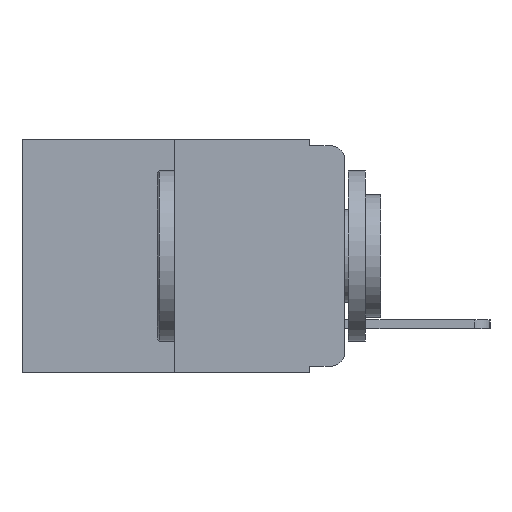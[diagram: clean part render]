
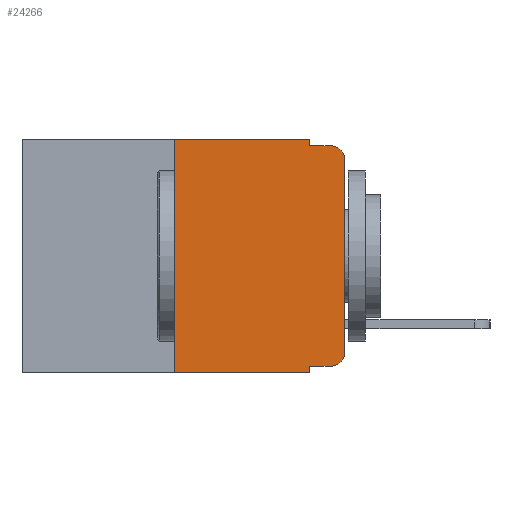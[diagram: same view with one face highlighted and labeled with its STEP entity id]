
A CAD part, left-side view. The second image highlights one B-rep face of the part: STEP entity #24266.
In plain terms, the highlighted planar face has unit normal (-1, 0, 0).
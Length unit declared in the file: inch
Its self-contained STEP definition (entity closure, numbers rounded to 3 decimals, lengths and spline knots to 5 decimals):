
#91 = DIRECTION ( 'NONE',  ( 0., 0., -1. ) ) ;
#935 = VERTEX_POINT ( 'NONE', #13057 ) ;
#1769 = CIRCLE ( 'NONE', #21188, 0.02 ) ;
#1805 = VERTEX_POINT ( 'NONE', #11658 ) ;
#1842 = CARTESIAN_POINT ( 'NONE',  ( 0., 0.051, 0. ) ) ;
#1958 = CARTESIAN_POINT ( 'NONE',  ( 0., 0., -0.03 ) ) ;
#2430 = CARTESIAN_POINT ( 'NONE',  ( 0., 0.473, 0. ) ) ;
#2524 = DIRECTION ( 'NONE',  ( -1., 0., 0. ) ) ;
#2760 = CARTESIAN_POINT ( 'NONE',  ( 0., 0.051, -0.343 ) ) ;
#3143 = CARTESIAN_POINT ( 'NONE',  ( 0., 0.25, -0.343 ) ) ;
#3428 = DIRECTION ( 'NONE',  ( 0., -1., 0. ) ) ;
#3642 = FACE_OUTER_BOUND ( 'NONE', #5323, .T. ) ;
#4246 = VECTOR ( 'NONE', #15215, 39.37008 ) ;
#4511 = VECTOR ( 'NONE', #8944, 39.37008 ) ;
#5126 = CARTESIAN_POINT ( 'NONE',  ( 0., 0.25, 0. ) ) ;
#5323 = EDGE_LOOP ( 'NONE', ( #5848, #6630, #7148, #7383, #7730, #7857, #8048, #8886, #10385, #14913 ) ) ;
#5848 = ORIENTED_EDGE ( 'NONE', *, *, #20655, .T. ) ;
#6630 = ORIENTED_EDGE ( 'NONE', *, *, #19411, .T. ) ;
#6721 = VERTEX_POINT ( 'NONE', #14300 ) ;
#6973 = VECTOR ( 'NONE', #20878, 39.37008 ) ;
#7148 = ORIENTED_EDGE ( 'NONE', *, *, #18197, .F. ) ;
#7259 = EDGE_CURVE ( 'NONE', #7272, #22454, #15063, .T. ) ;
#7272 = VERTEX_POINT ( 'NONE', #3143 ) ;
#7383 = ORIENTED_EDGE ( 'NONE', *, *, #15744, .F. ) ;
#7730 = ORIENTED_EDGE ( 'NONE', *, *, #13868, .F. ) ;
#7857 = ORIENTED_EDGE ( 'NONE', *, *, #14480, .F. ) ;
#7949 = AXIS2_PLACEMENT_3D ( 'NONE', #22651, #11613, #91 ) ;
#8048 = ORIENTED_EDGE ( 'NONE', *, *, #7259, .T. ) ;
#8066 = CARTESIAN_POINT ( 'NONE',  ( 0., 0., -0.313 ) ) ;
#8886 = ORIENTED_EDGE ( 'NONE', *, *, #13232, .F. ) ;
#8944 = DIRECTION ( 'NONE',  ( 0., 0., 1. ) ) ;
#9014 = VERTEX_POINT ( 'NONE', #8066 ) ;
#9462 = VERTEX_POINT ( 'NONE', #1958 ) ;
#9473 = EDGE_CURVE ( 'NONE', #12463, #9014, #19847, .T. ) ;
#9792 = CARTESIAN_POINT ( 'NONE',  ( 0., 0., 0. ) ) ;
#10176 = DIRECTION ( 'NONE',  ( 1., 0., 0. ) ) ;
#10378 = DIRECTION ( 'NONE',  ( 0., -1., 0. ) ) ;
#10385 = ORIENTED_EDGE ( 'NONE', *, *, #10762, .T. ) ;
#10762 = EDGE_CURVE ( 'NONE', #935, #12463, #19188, .T. ) ;
#11473 = CARTESIAN_POINT ( 'NONE',  ( 0., 0.473, 0. ) ) ;
#11613 = DIRECTION ( 'NONE',  ( -1., 0., 0. ) ) ;
#11658 = CARTESIAN_POINT ( 'NONE',  ( 0., 0.25, 0. ) ) ;
#12463 = VERTEX_POINT ( 'NONE', #14345 ) ;
#13057 = CARTESIAN_POINT ( 'NONE',  ( 0., 0.051, -0.333 ) ) ;
#13232 = EDGE_CURVE ( 'NONE', #935, #22454, #22925, .T. ) ;
#13436 = VERTEX_POINT ( 'NONE', #23091 ) ;
#13695 = VECTOR ( 'NONE', #17021, 39.37008 ) ;
#13868 = EDGE_CURVE ( 'NONE', #1805, #6721, #18611, .T. ) ;
#13925 = CARTESIAN_POINT ( 'NONE',  ( 0., 0.02, -0.03 ) ) ;
#14300 = CARTESIAN_POINT ( 'NONE',  ( 0., 0.051, 0. ) ) ;
#14345 = CARTESIAN_POINT ( 'NONE',  ( 0., 0.02, -0.333 ) ) ;
#14480 = EDGE_CURVE ( 'NONE', #7272, #1805, #19436, .T. ) ;
#14913 = ORIENTED_EDGE ( 'NONE', *, *, #9473, .T. ) ;
#15063 = LINE ( 'NONE', #23272, #19374 ) ;
#15215 = DIRECTION ( 'NONE',  ( 0., -1., 0. ) ) ;
#15744 = EDGE_CURVE ( 'NONE', #6721, #13436, #21656, .T. ) ;
#15809 = DIRECTION ( 'NONE',  ( 0., 0., -1. ) ) ;
#16168 = DIRECTION ( 'NONE',  ( 0., 0., -1. ) ) ;
#16659 = CARTESIAN_POINT ( 'NONE',  ( 0., 0.051, -0.01 ) ) ;
#17021 = DIRECTION ( 'NONE',  ( 0., 0., -1. ) ) ;
#17603 = CARTESIAN_POINT ( 'NONE',  ( 0., 0.02, -0.01 ) ) ;
#17934 = VECTOR ( 'NONE', #16168, 39.37008 ) ;
#18012 = CARTESIAN_POINT ( 'NONE',  ( 0., 0.051, 0. ) ) ;
#18052 = VECTOR ( 'NONE', #22502, 39.37008 ) ;
#18197 = EDGE_CURVE ( 'NONE', #13436, #18527, #19541, .T. ) ;
#18527 = VERTEX_POINT ( 'NONE', #17603 ) ;
#18611 = LINE ( 'NONE', #11473, #18052 ) ;
#18990 = AXIS2_PLACEMENT_3D ( 'NONE', #2430, #10176, #23079 ) ;
#19188 = LINE ( 'NONE', #22514, #4246 ) ;
#19374 = VECTOR ( 'NONE', #10378, 39.37008 ) ;
#19411 = EDGE_CURVE ( 'NONE', #9462, #18527, #1769, .T. ) ;
#19436 = LINE ( 'NONE', #5126, #4511 ) ;
#19541 = LINE ( 'NONE', #16659, #20119 ) ;
#19847 = CIRCLE ( 'NONE', #7949, 0.02 ) ;
#20119 = VECTOR ( 'NONE', #3428, 39.37008 ) ;
#20655 = EDGE_CURVE ( 'NONE', #9014, #9462, #21816, .T. ) ;
#20878 = DIRECTION ( 'NONE',  ( 0., 0., 1. ) ) ;
#21188 = AXIS2_PLACEMENT_3D ( 'NONE', #13925, #2524, #15809 ) ;
#21243 = PLANE ( 'NONE',  #18990 ) ;
#21656 = LINE ( 'NONE', #18012, #17934 ) ;
#21816 = LINE ( 'NONE', #9792, #6973 ) ;
#22454 = VERTEX_POINT ( 'NONE', #2760 ) ;
#22502 = DIRECTION ( 'NONE',  ( 0., -1., 0. ) ) ;
#22514 = CARTESIAN_POINT ( 'NONE',  ( 0., 0.051, -0.333 ) ) ;
#22651 = CARTESIAN_POINT ( 'NONE',  ( 0., 0.02, -0.313 ) ) ;
#22925 = LINE ( 'NONE', #1842, #13695 ) ;
#23079 = DIRECTION ( 'NONE',  ( 0., 0., -1. ) ) ;
#23091 = CARTESIAN_POINT ( 'NONE',  ( 0., 0.051, -0.01 ) ) ;
#23272 = CARTESIAN_POINT ( 'NONE',  ( 0., 0.473, -0.343 ) ) ;
#24266 = ADVANCED_FACE ( 'NONE', ( #3642 ), #21243, .F. ) ;
